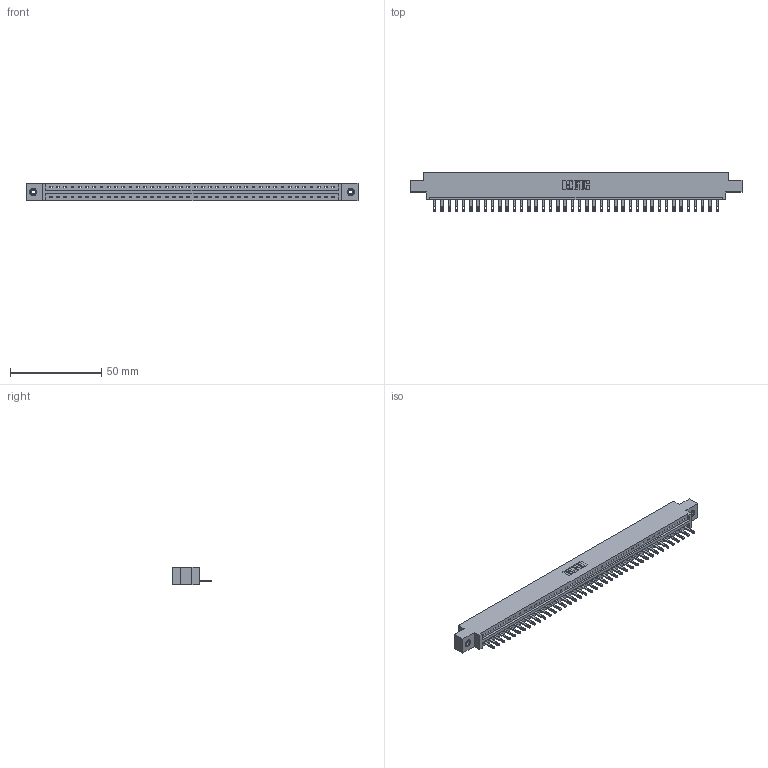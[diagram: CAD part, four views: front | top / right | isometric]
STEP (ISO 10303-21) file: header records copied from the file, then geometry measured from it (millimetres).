
FILE_DESCRIPTION (( 'STEP AP203' ), '1' );
FILE_NAME ('887-040-500-608.STEP', '2020-09-20T23:30:11', ( '' ), ( '' ), 'SwSTEP 2.0', 'SolidWorks 2020', '' );
FILE_SCHEMA (( 'CONFIG_CONTROL_DESIGN' ));
Length unit declared in the file: inch
Products named in the file (4): 345-250-001_345-250-003-102; 837 Part_0.170 Offset - 0.156 Dia-TI; 345-292-001_345-293-100; 887-040-500-608
Assembly tree (43 placements, depth 2):
  887-040-500-608
    837 Part_0.170 Offset - 0.156 Dia-TI
    345-292-001_345-293-100  x40
    345-250-001_345-250-003-102  x2
Bounding box: 181.51 x 21.85 x 9.4 mm (x, y, z)
Volume: 18740.5 mm3; surface area: 19573.9 mm2
Topology: 43 solids, 43 shells, 2498 faces, 7659 edges, 5098 vertices
Faces by surface type: plane 1706, cylinder 776, cone 12, torus 4
Entity records: 31240 total; most frequent: CARTESIAN_POINT 5421, ORIENTED_EDGE 5390, DIRECTION 4601, EDGE_CURVE 2695, LINE 2543, VECTOR 2543, VERTEX_POINT 1792, AXIS2_PLACEMENT_3D 1029
